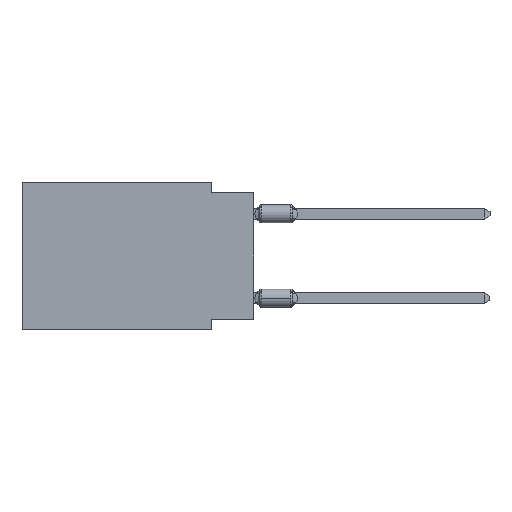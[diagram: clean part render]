
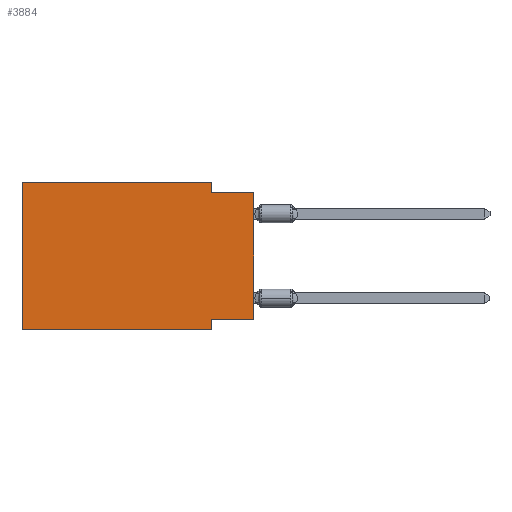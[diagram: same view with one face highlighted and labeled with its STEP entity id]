
A CAD part, left-side view. The second image highlights one B-rep face of the part: STEP entity #3884.
In plain terms, the highlighted planar face has unit normal (-1, 0, 0).
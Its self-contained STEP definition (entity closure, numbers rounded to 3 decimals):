
#161 = VECTOR ( 'NONE', #1637, 1000. ) ;
#240 = ORIENTED_EDGE ( 'NONE', *, *, #13446, .F. ) ;
#345 = VECTOR ( 'NONE', #2395, 1000. ) ;
#743 = LINE ( 'NONE', #10420, #2789 ) ;
#977 = CARTESIAN_POINT ( 'NONE',  ( 0., 0., -8.255 ) ) ;
#1141 = DIRECTION ( 'NONE',  ( 0., 0., -1. ) ) ;
#1532 = ORIENTED_EDGE ( 'NONE', *, *, #2312, .F. ) ;
#1558 = LINE ( 'NONE', #12000, #11722 ) ;
#1569 = CARTESIAN_POINT ( 'NONE',  ( 0., 2.54, 0. ) ) ;
#1587 = EDGE_CURVE ( 'NONE', #7849, #9713, #5355, .T. ) ;
#1637 = DIRECTION ( 'NONE',  ( 0., 0., -1. ) ) ;
#1778 = CARTESIAN_POINT ( 'NONE',  ( 0., 0., -0.635 ) ) ;
#2297 = EDGE_CURVE ( 'NONE', #2502, #4499, #10690, .T. ) ;
#2312 = EDGE_CURVE ( 'NONE', #8607, #11056, #2504, .T. ) ;
#2395 = DIRECTION ( 'NONE',  ( 0., -1., 0. ) ) ;
#2502 = VERTEX_POINT ( 'NONE', #6897 ) ;
#2504 = LINE ( 'NONE', #6761, #13119 ) ;
#2789 = VECTOR ( 'NONE', #10358, 1000. ) ;
#2912 = ORIENTED_EDGE ( 'NONE', *, *, #2297, .F. ) ;
#2976 = DIRECTION ( 'NONE',  ( 0., 1., 0. ) ) ;
#3017 = LINE ( 'NONE', #12563, #5024 ) ;
#3223 = CARTESIAN_POINT ( 'NONE',  ( 0., 0., -0.635 ) ) ;
#3324 = CARTESIAN_POINT ( 'NONE',  ( 0., 0., -8.255 ) ) ;
#3340 = EDGE_CURVE ( 'NONE', #12420, #4499, #3017, .T. ) ;
#3402 = CARTESIAN_POINT ( 'NONE',  ( 0., 13.97, 0. ) ) ;
#3772 = LINE ( 'NONE', #1569, #161 ) ;
#3884 = ADVANCED_FACE ( 'NONE', ( #6356 ), #10556, .F. ) ;
#4499 = VERTEX_POINT ( 'NONE', #13395 ) ;
#4516 = ORIENTED_EDGE ( 'NONE', *, *, #3340, .T. ) ;
#4789 = VECTOR ( 'NONE', #7597, 1000. ) ;
#5024 = VECTOR ( 'NONE', #9344, 1000. ) ;
#5355 = LINE ( 'NONE', #3223, #345 ) ;
#5918 = VERTEX_POINT ( 'NONE', #3324 ) ;
#6334 = EDGE_LOOP ( 'NONE', ( #12091, #10687, #9006, #1532, #240, #4516, #2912, #6511 ) ) ;
#6356 = FACE_OUTER_BOUND ( 'NONE', #6334, .T. ) ;
#6511 = ORIENTED_EDGE ( 'NONE', *, *, #8990, .F. ) ;
#6761 = CARTESIAN_POINT ( 'NONE',  ( 0., 13.97, 0. ) ) ;
#6897 = CARTESIAN_POINT ( 'NONE',  ( 0., 2.54, -8.255 ) ) ;
#7597 = DIRECTION ( 'NONE',  ( 0., 0., -1. ) ) ;
#7600 = DIRECTION ( 'NONE',  ( 1., 0., 0. ) ) ;
#7735 = CARTESIAN_POINT ( 'NONE',  ( 0., 2.54, -8.89 ) ) ;
#7849 = VERTEX_POINT ( 'NONE', #9554 ) ;
#8207 = LINE ( 'NONE', #977, #9931 ) ;
#8607 = VERTEX_POINT ( 'NONE', #10476 ) ;
#8990 = EDGE_CURVE ( 'NONE', #5918, #2502, #8207, .T. ) ;
#9006 = ORIENTED_EDGE ( 'NONE', *, *, #13302, .F. ) ;
#9344 = DIRECTION ( 'NONE',  ( 0., -1., 0. ) ) ;
#9554 = CARTESIAN_POINT ( 'NONE',  ( 0., 2.54, -0.635 ) ) ;
#9713 = VERTEX_POINT ( 'NONE', #1778 ) ;
#9921 = EDGE_CURVE ( 'NONE', #5918, #9713, #1558, .T. ) ;
#9931 = VECTOR ( 'NONE', #2976, 1000. ) ;
#10252 = CARTESIAN_POINT ( 'NONE',  ( 0., 2.54, 0. ) ) ;
#10358 = DIRECTION ( 'NONE',  ( 0., 0., 1. ) ) ;
#10420 = CARTESIAN_POINT ( 'NONE',  ( 0., 13.97, 0. ) ) ;
#10476 = CARTESIAN_POINT ( 'NONE',  ( 0., 13.97, 0. ) ) ;
#10556 = PLANE ( 'NONE',  #11802 ) ;
#10687 = ORIENTED_EDGE ( 'NONE', *, *, #1587, .F. ) ;
#10690 = LINE ( 'NONE', #7735, #4789 ) ;
#10854 = CARTESIAN_POINT ( 'NONE',  ( 0., 13.97, -8.89 ) ) ;
#11056 = VERTEX_POINT ( 'NONE', #10252 ) ;
#11722 = VECTOR ( 'NONE', #11933, 1000. ) ;
#11802 = AXIS2_PLACEMENT_3D ( 'NONE', #3402, #7600, #1141 ) ;
#11933 = DIRECTION ( 'NONE',  ( 0., 0., 1. ) ) ;
#12000 = CARTESIAN_POINT ( 'NONE',  ( 0., 0., 0. ) ) ;
#12091 = ORIENTED_EDGE ( 'NONE', *, *, #9921, .T. ) ;
#12420 = VERTEX_POINT ( 'NONE', #10854 ) ;
#12563 = CARTESIAN_POINT ( 'NONE',  ( 0., 13.97, -8.89 ) ) ;
#13014 = DIRECTION ( 'NONE',  ( 0., -1., 0. ) ) ;
#13119 = VECTOR ( 'NONE', #13014, 1000. ) ;
#13302 = EDGE_CURVE ( 'NONE', #11056, #7849, #3772, .T. ) ;
#13395 = CARTESIAN_POINT ( 'NONE',  ( 0., 2.54, -8.89 ) ) ;
#13446 = EDGE_CURVE ( 'NONE', #12420, #8607, #743, .T. ) ;
